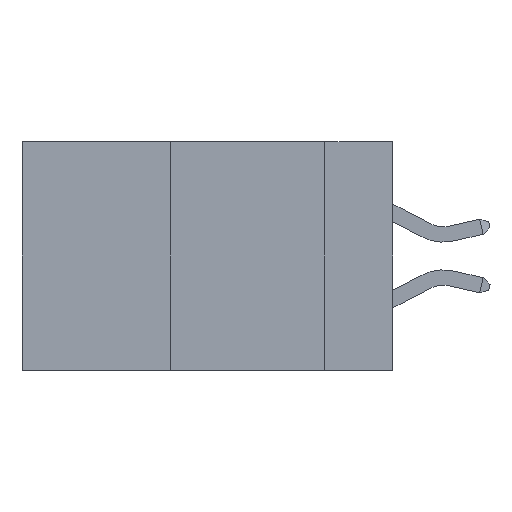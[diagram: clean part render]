
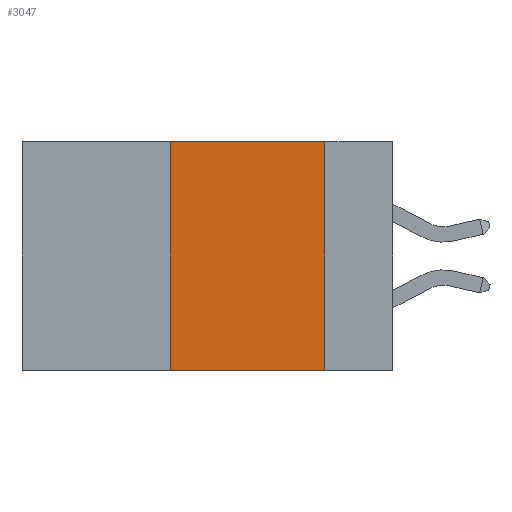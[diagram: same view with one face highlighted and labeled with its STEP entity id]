
A CAD part, left-side view. The second image highlights one B-rep face of the part: STEP entity #3047.
In plain terms, the highlighted planar face has unit normal (-1, 0, 0).
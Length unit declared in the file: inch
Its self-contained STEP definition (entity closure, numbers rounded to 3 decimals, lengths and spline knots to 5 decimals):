
#438 = DIRECTION ( 'NONE',  ( 0., 0., -1. ) ) ;
#482 = DIRECTION ( 'NONE',  ( 0., 0., 1. ) ) ;
#973 = VECTOR ( 'NONE', #7319, 39.37008 ) ;
#1061 = VERTEX_POINT ( 'NONE', #16394 ) ;
#1461 = LINE ( 'NONE', #9400, #6806 ) ;
#2930 = CARTESIAN_POINT ( 'NONE',  ( 0., 0.6, 0. ) ) ;
#3047 = ADVANCED_FACE ( 'NONE', ( #6248 ), #8668, .F. ) ;
#5112 = VERTEX_POINT ( 'NONE', #15798 ) ;
#5326 = CARTESIAN_POINT ( 'NONE',  ( 0., 0.11, 0. ) ) ;
#5342 = VERTEX_POINT ( 'NONE', #16426 ) ;
#5581 = EDGE_CURVE ( 'NONE', #8640, #1061, #7392, .T. ) ;
#5723 = LINE ( 'NONE', #2930, #9950 ) ;
#5853 = EDGE_CURVE ( 'NONE', #5342, #8640, #5723, .T. ) ;
#6248 = FACE_OUTER_BOUND ( 'NONE', #6946, .T. ) ;
#6806 = VECTOR ( 'NONE', #9458, 39.37008 ) ;
#6946 = EDGE_LOOP ( 'NONE', ( #13493, #10177, #15087, #8010 ) ) ;
#7319 = DIRECTION ( 'NONE',  ( 0., 0., -1. ) ) ;
#7392 = LINE ( 'NONE', #15437, #973 ) ;
#7479 = CARTESIAN_POINT ( 'NONE',  ( 0., 0.6, 0. ) ) ;
#7514 = LINE ( 'NONE', #9910, #10287 ) ;
#8010 = ORIENTED_EDGE ( 'NONE', *, *, #10667, .T. ) ;
#8447 = EDGE_CURVE ( 'NONE', #5112, #5342, #7514, .T. ) ;
#8612 = DIRECTION ( 'NONE',  ( 1., 0., 0. ) ) ;
#8640 = VERTEX_POINT ( 'NONE', #5326 ) ;
#8668 = PLANE ( 'NONE',  #11845 ) ;
#9400 = CARTESIAN_POINT ( 'NONE',  ( 0., 0.6, -0.37 ) ) ;
#9458 = DIRECTION ( 'NONE',  ( 0., -1., 0. ) ) ;
#9910 = CARTESIAN_POINT ( 'NONE',  ( 0., 0.36, 0. ) ) ;
#9950 = VECTOR ( 'NONE', #12422, 39.37008 ) ;
#10177 = ORIENTED_EDGE ( 'NONE', *, *, #5853, .F. ) ;
#10287 = VECTOR ( 'NONE', #482, 39.37008 ) ;
#10667 = EDGE_CURVE ( 'NONE', #5112, #1061, #1461, .T. ) ;
#11845 = AXIS2_PLACEMENT_3D ( 'NONE', #7479, #8612, #438 ) ;
#12422 = DIRECTION ( 'NONE',  ( 0., -1., 0. ) ) ;
#13493 = ORIENTED_EDGE ( 'NONE', *, *, #5581, .F. ) ;
#15087 = ORIENTED_EDGE ( 'NONE', *, *, #8447, .F. ) ;
#15437 = CARTESIAN_POINT ( 'NONE',  ( 0., 0.11, 0. ) ) ;
#15798 = CARTESIAN_POINT ( 'NONE',  ( 0., 0.36, -0.37 ) ) ;
#16394 = CARTESIAN_POINT ( 'NONE',  ( 0., 0.11, -0.37 ) ) ;
#16426 = CARTESIAN_POINT ( 'NONE',  ( 0., 0.36, 0. ) ) ;
